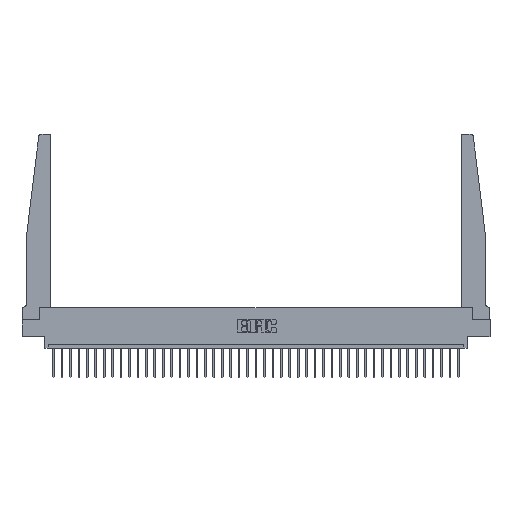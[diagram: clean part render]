
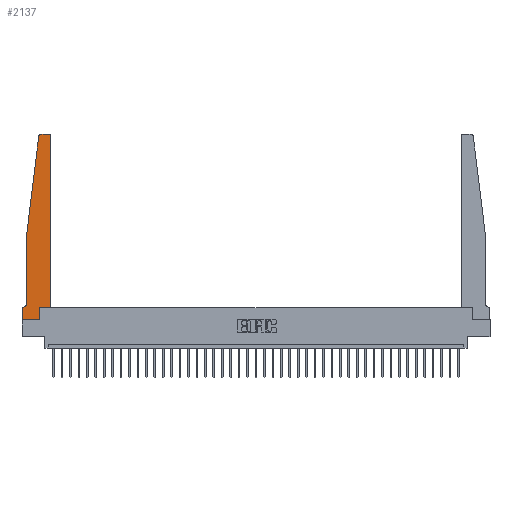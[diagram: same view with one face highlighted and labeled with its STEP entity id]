
A CAD part, top view. The second image highlights one B-rep face of the part: STEP entity #2137.
In plain terms, the highlighted planar face has unit normal (0, 0, 1).
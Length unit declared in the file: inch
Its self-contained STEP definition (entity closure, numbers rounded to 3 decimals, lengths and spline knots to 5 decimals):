
#812 = LINE ( 'NONE', #8362, #923 ) ;
#901 = LINE ( 'NONE', #30494, #8974 ) ;
#923 = VECTOR ( 'NONE', #30052, 39.37008 ) ;
#1161 = CARTESIAN_POINT ( 'NONE',  ( 0.395, 2.72, 0.37 ) ) ;
#2137 = ADVANCED_FACE ( 'NONE', ( #17706 ), #6830, .T. ) ;
#2452 = DIRECTION ( 'NONE',  ( 0., 0., 1. ) ) ;
#2611 = EDGE_CURVE ( 'NONE', #16376, #25188, #13235, .T. ) ;
#2761 = AXIS2_PLACEMENT_3D ( 'NONE', #6903, #12174, #31050 ) ;
#2895 = CIRCLE ( 'NONE', #4028, 0.03 ) ;
#4028 = AXIS2_PLACEMENT_3D ( 'NONE', #1161, #28092, #33221 ) ;
#4492 = VECTOR ( 'NONE', #18118, 39.37008 ) ;
#5623 = CARTESIAN_POINT ( 'NONE',  ( 0.27653, 2.72, 0.37 ) ) ;
#6180 = CARTESIAN_POINT ( 'NONE',  ( 0.065, 1.25, 0.37 ) ) ;
#6830 = PLANE ( 'NONE',  #8877 ) ;
#6866 = CARTESIAN_POINT ( 'NONE',  ( 0.065, 1.25, 0.37 ) ) ;
#6903 = CARTESIAN_POINT ( 'NONE',  ( 0.015, 0.2375, 0.37 ) ) ;
#7524 = EDGE_CURVE ( 'NONE', #31734, #22366, #2895, .T. ) ;
#8227 = VECTOR ( 'NONE', #30497, 39.37008 ) ;
#8322 = CARTESIAN_POINT ( 'NONE',  ( 0.24675, 2.72367, 0.37 ) ) ;
#8362 = CARTESIAN_POINT ( 'NONE',  ( 0.065, 0.1875, 0.37 ) ) ;
#8877 = AXIS2_PLACEMENT_3D ( 'NONE', #33965, #25851, #10158 ) ;
#8974 = VECTOR ( 'NONE', #16912, 39.37008 ) ;
#9366 = ORIENTED_EDGE ( 'NONE', *, *, #2611, .T. ) ;
#10158 = DIRECTION ( 'NONE',  ( 1., 0., 0. ) ) ;
#10272 = LINE ( 'NONE', #12197, #17831 ) ;
#10491 = CARTESIAN_POINT ( 'NONE',  ( 0.2605, 0., 0.37 ) ) ;
#11291 = CARTESIAN_POINT ( 'NONE',  ( 0.25, 2.75, 0.37 ) ) ;
#11783 = VERTEX_POINT ( 'NONE', #10491 ) ;
#12174 = DIRECTION ( 'NONE',  ( 0., 0., -1. ) ) ;
#12197 = CARTESIAN_POINT ( 'NONE',  ( 0., 0., 0.37 ) ) ;
#12263 = VECTOR ( 'NONE', #14777, 39.37008 ) ;
#12477 = ORIENTED_EDGE ( 'NONE', *, *, #15620, .T. ) ;
#12990 = ORIENTED_EDGE ( 'NONE', *, *, #25709, .T. ) ;
#13235 = LINE ( 'NONE', #21002, #22922 ) ;
#13334 = ORIENTED_EDGE ( 'NONE', *, *, #33161, .T. ) ;
#13489 = VECTOR ( 'NONE', #30483, 39.37008 ) ;
#13519 = CARTESIAN_POINT ( 'NONE',  ( 0.395, 2.75, 0.37 ) ) ;
#13855 = VERTEX_POINT ( 'NONE', #25261 ) ;
#14101 = LINE ( 'NONE', #11291, #13489 ) ;
#14777 = DIRECTION ( 'NONE',  ( 0., 1., 0. ) ) ;
#15523 = CIRCLE ( 'NONE', #30168, 0.03 ) ;
#15620 = EDGE_CURVE ( 'NONE', #28863, #16376, #15523, .T. ) ;
#15631 = CARTESIAN_POINT ( 'NONE',  ( 0., 0.1875, 0.37 ) ) ;
#15716 = DIRECTION ( 'NONE',  ( -0.122, -0.992, 0. ) ) ;
#15759 = CARTESIAN_POINT ( 'NONE',  ( 0.425, 2.72, 0.37 ) ) ;
#15967 = EDGE_CURVE ( 'NONE', #27374, #31290, #812, .T. ) ;
#16376 = VERTEX_POINT ( 'NONE', #8322 ) ;
#16912 = DIRECTION ( 'NONE',  ( 1., 0., 0. ) ) ;
#17529 = CARTESIAN_POINT ( 'NONE',  ( 0.2605, 0.18, 0.37 ) ) ;
#17706 = FACE_OUTER_BOUND ( 'NONE', #24595, .T. ) ;
#17831 = VECTOR ( 'NONE', #21020, 39.37008 ) ;
#17869 = EDGE_CURVE ( 'NONE', #11783, #26944, #23242, .T. ) ;
#18012 = ORIENTED_EDGE ( 'NONE', *, *, #17869, .T. ) ;
#18118 = DIRECTION ( 'NONE',  ( 0., -1., 0. ) ) ;
#18644 = DIRECTION ( 'NONE',  ( 1., 0., 0. ) ) ;
#18703 = CARTESIAN_POINT ( 'NONE',  ( 0.27653, 2.75, 0.37 ) ) ;
#19299 = EDGE_CURVE ( 'NONE', #31290, #25743, #34559, .T. ) ;
#19749 = ORIENTED_EDGE ( 'NONE', *, *, #29461, .T. ) ;
#20424 = CARTESIAN_POINT ( 'NONE',  ( 0.425, 0.18, 0.37 ) ) ;
#21002 = CARTESIAN_POINT ( 'NONE',  ( 0.065, 1.25, 0.37 ) ) ;
#21020 = DIRECTION ( 'NONE',  ( 1., 0., 0. ) ) ;
#22221 = DIRECTION ( 'NONE',  ( 0., -1., 0. ) ) ;
#22366 = VERTEX_POINT ( 'NONE', #13519 ) ;
#22922 = VECTOR ( 'NONE', #15716, 39.37008 ) ;
#23242 = LINE ( 'NONE', #30813, #12263 ) ;
#23332 = CARTESIAN_POINT ( 'NONE',  ( 0., 0., 0.37 ) ) ;
#23856 = VERTEX_POINT ( 'NONE', #24329 ) ;
#24329 = CARTESIAN_POINT ( 'NONE',  ( 0.065, 0.2375, 0.37 ) ) ;
#24595 = EDGE_LOOP ( 'NONE', ( #33667, #12477, #9366, #33061, #32328, #27079, #30092, #12990, #18012, #19749, #13334, #30808 ) ) ;
#24754 = VECTOR ( 'NONE', #22221, 39.37008 ) ;
#25188 = VERTEX_POINT ( 'NONE', #6866 ) ;
#25261 = CARTESIAN_POINT ( 'NONE',  ( 0.425, 0.18, 0.37 ) ) ;
#25709 = EDGE_CURVE ( 'NONE', #25743, #11783, #10272, .T. ) ;
#25743 = VERTEX_POINT ( 'NONE', #23332 ) ;
#25851 = DIRECTION ( 'NONE',  ( 0., 0., 1. ) ) ;
#26944 = VERTEX_POINT ( 'NONE', #17529 ) ;
#27079 = ORIENTED_EDGE ( 'NONE', *, *, #15967, .T. ) ;
#27374 = VERTEX_POINT ( 'NONE', #33383 ) ;
#27655 = EDGE_CURVE ( 'NONE', #22366, #28863, #14101, .T. ) ;
#28092 = DIRECTION ( 'NONE',  ( 0., 0., 1. ) ) ;
#28863 = VERTEX_POINT ( 'NONE', #18703 ) ;
#29209 = EDGE_CURVE ( 'NONE', #23856, #27374, #33750, .T. ) ;
#29454 = EDGE_CURVE ( 'NONE', #25188, #23856, #30319, .T. ) ;
#29461 = EDGE_CURVE ( 'NONE', #26944, #13855, #901, .T. ) ;
#30052 = DIRECTION ( 'NONE',  ( -1., 0., 0. ) ) ;
#30092 = ORIENTED_EDGE ( 'NONE', *, *, #19299, .T. ) ;
#30168 = AXIS2_PLACEMENT_3D ( 'NONE', #5623, #2452, #18644 ) ;
#30319 = LINE ( 'NONE', #6180, #24754 ) ;
#30483 = DIRECTION ( 'NONE',  ( -1., 0., 0. ) ) ;
#30494 = CARTESIAN_POINT ( 'NONE',  ( 0.425, 0.18, 0.37 ) ) ;
#30497 = DIRECTION ( 'NONE',  ( 0., 1., 0. ) ) ;
#30808 = ORIENTED_EDGE ( 'NONE', *, *, #7524, .T. ) ;
#30813 = CARTESIAN_POINT ( 'NONE',  ( 0.2605, 0.18, 0.37 ) ) ;
#31050 = DIRECTION ( 'NONE',  ( -1., 0., 0. ) ) ;
#31290 = VERTEX_POINT ( 'NONE', #15631 ) ;
#31734 = VERTEX_POINT ( 'NONE', #15759 ) ;
#32328 = ORIENTED_EDGE ( 'NONE', *, *, #29209, .T. ) ;
#33061 = ORIENTED_EDGE ( 'NONE', *, *, #29454, .T. ) ;
#33161 = EDGE_CURVE ( 'NONE', #13855, #31734, #33647, .T. ) ;
#33221 = DIRECTION ( 'NONE',  ( 1., 0., 0. ) ) ;
#33383 = CARTESIAN_POINT ( 'NONE',  ( 0.015, 0.1875, 0.37 ) ) ;
#33647 = LINE ( 'NONE', #20424, #8227 ) ;
#33667 = ORIENTED_EDGE ( 'NONE', *, *, #27655, .T. ) ;
#33750 = CIRCLE ( 'NONE', #2761, 0.05 ) ;
#33965 = CARTESIAN_POINT ( 'NONE',  ( 0., 0.1875, 0.37 ) ) ;
#34032 = CARTESIAN_POINT ( 'NONE',  ( 0., 0., 0.37 ) ) ;
#34559 = LINE ( 'NONE', #34032, #4492 ) ;
